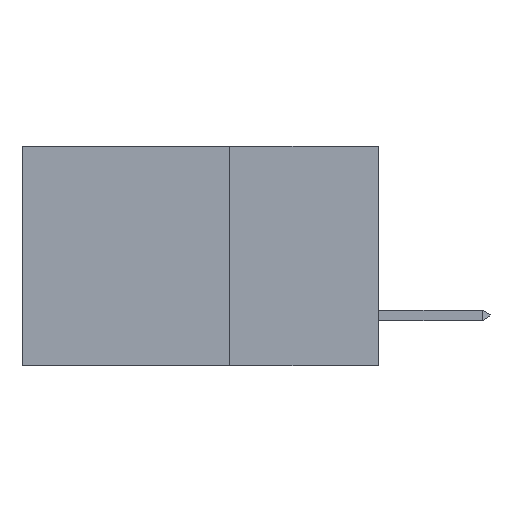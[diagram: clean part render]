
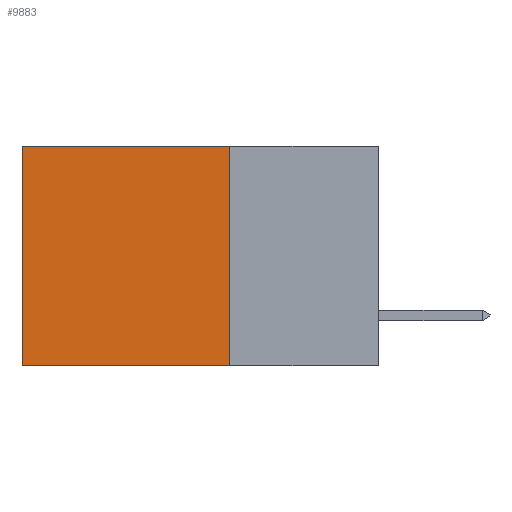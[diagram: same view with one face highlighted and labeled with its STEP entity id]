
A CAD part, left-side view. The second image highlights one B-rep face of the part: STEP entity #9883.
In plain terms, the highlighted planar face has unit normal (-1, 0, 0).
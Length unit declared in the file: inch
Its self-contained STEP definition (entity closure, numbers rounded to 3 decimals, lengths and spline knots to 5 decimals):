
#324 = EDGE_LOOP ( 'NONE', ( #1260, #4187, #8068, #9390 ) ) ;
#385 = VERTEX_POINT ( 'NONE', #2106 ) ;
#420 = VERTEX_POINT ( 'NONE', #3178 ) ;
#444 = VERTEX_POINT ( 'NONE', #9234 ) ;
#830 = LINE ( 'NONE', #11983, #9199 ) ;
#1066 = DIRECTION ( 'NONE',  ( 0., 0., -1. ) ) ;
#1260 = ORIENTED_EDGE ( 'NONE', *, *, #3559, .T. ) ;
#1917 = LINE ( 'NONE', #10514, #4753 ) ;
#2106 = CARTESIAN_POINT ( 'NONE',  ( 0.2615, 0.6, 0. ) ) ;
#2831 = VECTOR ( 'NONE', #6714, 39.37008 ) ;
#3178 = CARTESIAN_POINT ( 'NONE',  ( 0.2615, 0.6, -0.37 ) ) ;
#3241 = AXIS2_PLACEMENT_3D ( 'NONE', #3621, #8368, #7244 ) ;
#3559 = EDGE_CURVE ( 'NONE', #385, #420, #830, .T. ) ;
#3621 = CARTESIAN_POINT ( 'NONE',  ( 0.2615, 0.25, -0.37 ) ) ;
#3911 = LINE ( 'NONE', #7675, #2831 ) ;
#4187 = ORIENTED_EDGE ( 'NONE', *, *, #9429, .F. ) ;
#4753 = VECTOR ( 'NONE', #1066, 39.37008 ) ;
#5345 = FACE_OUTER_BOUND ( 'NONE', #324, .T. ) ;
#5602 = VERTEX_POINT ( 'NONE', #9061 ) ;
#6714 = DIRECTION ( 'NONE',  ( 0., 1., 0. ) ) ;
#7244 = DIRECTION ( 'NONE',  ( 0., 0., -1. ) ) ;
#7296 = LINE ( 'NONE', #10139, #10243 ) ;
#7675 = CARTESIAN_POINT ( 'NONE',  ( 0.2615, 0.25, -0.37 ) ) ;
#8068 = ORIENTED_EDGE ( 'NONE', *, *, #10050, .F. ) ;
#8118 = PLANE ( 'NONE',  #3241 ) ;
#8368 = DIRECTION ( 'NONE',  ( 1., 0., 0. ) ) ;
#9061 = CARTESIAN_POINT ( 'NONE',  ( 0.2615, 0.25, -0.37 ) ) ;
#9152 = DIRECTION ( 'NONE',  ( 0., 1., 0. ) ) ;
#9199 = VECTOR ( 'NONE', #11043, 39.37008 ) ;
#9234 = CARTESIAN_POINT ( 'NONE',  ( 0.2615, 0.25, 0. ) ) ;
#9390 = ORIENTED_EDGE ( 'NONE', *, *, #10314, .T. ) ;
#9429 = EDGE_CURVE ( 'NONE', #5602, #420, #3911, .T. ) ;
#9883 = ADVANCED_FACE ( 'NONE', ( #5345 ), #8118, .F. ) ;
#10050 = EDGE_CURVE ( 'NONE', #444, #5602, #1917, .T. ) ;
#10139 = CARTESIAN_POINT ( 'NONE',  ( 0.2615, 0.25, 0. ) ) ;
#10243 = VECTOR ( 'NONE', #9152, 39.37008 ) ;
#10314 = EDGE_CURVE ( 'NONE', #444, #385, #7296, .T. ) ;
#10514 = CARTESIAN_POINT ( 'NONE',  ( 0.2615, 0.25, -0.37 ) ) ;
#11043 = DIRECTION ( 'NONE',  ( 0., 0., -1. ) ) ;
#11983 = CARTESIAN_POINT ( 'NONE',  ( 0.2615, 0.6, -0.37 ) ) ;
